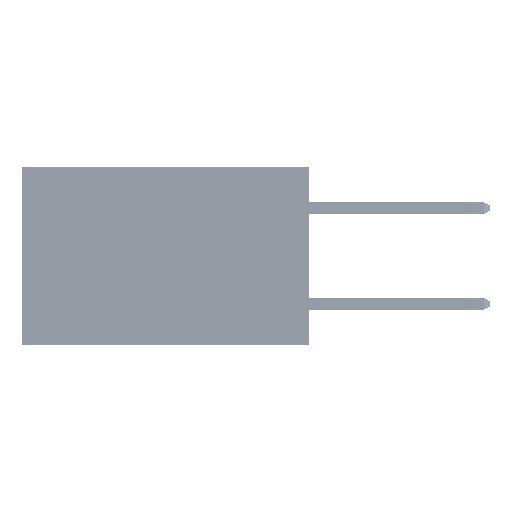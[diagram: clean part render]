
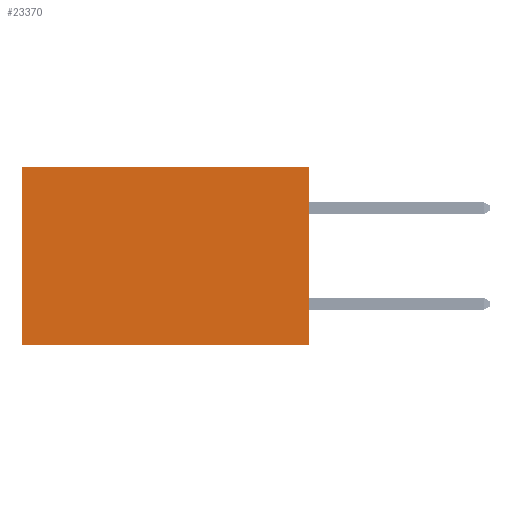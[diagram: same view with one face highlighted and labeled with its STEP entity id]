
A CAD part, left-side view. The second image highlights one B-rep face of the part: STEP entity #23370.
In plain terms, the highlighted planar face has unit normal (-1, 0, 0).
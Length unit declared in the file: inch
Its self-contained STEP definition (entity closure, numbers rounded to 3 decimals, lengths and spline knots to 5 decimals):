
#3877 = CARTESIAN_POINT ( 'NONE',  ( 0.2875, 0., 0. ) ) ;
#4240 = EDGE_CURVE ( 'NONE', #31126, #8284, #42876, .T. ) ;
#6278 = ORIENTED_EDGE ( 'NONE', *, *, #15349, .F. ) ;
#8284 = VERTEX_POINT ( 'NONE', #21485 ) ;
#8937 = VERTEX_POINT ( 'NONE', #30528 ) ;
#10186 = EDGE_LOOP ( 'NONE', ( #36949, #6278, #23037, #30390 ) ) ;
#10189 = CARTESIAN_POINT ( 'NONE',  ( 0.2875, 0.6, 0. ) ) ;
#12075 = AXIS2_PLACEMENT_3D ( 'NONE', #41348, #17093, #37240 ) ;
#12140 = VECTOR ( 'NONE', #31853, 39.37008 ) ;
#14491 = VECTOR ( 'NONE', #31919, 39.37008 ) ;
#15349 = EDGE_CURVE ( 'NONE', #8284, #30397, #39154, .T. ) ;
#16026 = CARTESIAN_POINT ( 'NONE',  ( 0.2875, 0., 0. ) ) ;
#17093 = DIRECTION ( 'NONE',  ( 1., 0., 0. ) ) ;
#17377 = VECTOR ( 'NONE', #38400, 39.37008 ) ;
#19308 = DIRECTION ( 'NONE',  ( 0., 0., -1. ) ) ;
#21485 = CARTESIAN_POINT ( 'NONE',  ( 0.2875, 0., -0.37 ) ) ;
#23037 = ORIENTED_EDGE ( 'NONE', *, *, #4240, .F. ) ;
#23370 = ADVANCED_FACE ( 'NONE', ( #31861 ), #48587, .F. ) ;
#27455 = CARTESIAN_POINT ( 'NONE',  ( 0.2875, 0.6, -0.37 ) ) ;
#28071 = LINE ( 'NONE', #3877, #12140 ) ;
#29906 = EDGE_CURVE ( 'NONE', #31126, #8937, #28071, .T. ) ;
#30390 = ORIENTED_EDGE ( 'NONE', *, *, #29906, .T. ) ;
#30397 = VERTEX_POINT ( 'NONE', #27455 ) ;
#30528 = CARTESIAN_POINT ( 'NONE',  ( 0.2875, 0.6, 0. ) ) ;
#31126 = VERTEX_POINT ( 'NONE', #16026 ) ;
#31853 = DIRECTION ( 'NONE',  ( 0., 1., 0. ) ) ;
#31861 = FACE_OUTER_BOUND ( 'NONE', #10186, .T. ) ;
#31919 = DIRECTION ( 'NONE',  ( 0., 1., 0. ) ) ;
#34276 = VECTOR ( 'NONE', #19308, 39.37008 ) ;
#34912 = EDGE_CURVE ( 'NONE', #8937, #30397, #49419, .T. ) ;
#36949 = ORIENTED_EDGE ( 'NONE', *, *, #34912, .T. ) ;
#37240 = DIRECTION ( 'NONE',  ( 0., 0., -1. ) ) ;
#38400 = DIRECTION ( 'NONE',  ( 0., 0., -1. ) ) ;
#39154 = LINE ( 'NONE', #39703, #14491 ) ;
#39703 = CARTESIAN_POINT ( 'NONE',  ( 0.2875, 0., -0.37 ) ) ;
#41348 = CARTESIAN_POINT ( 'NONE',  ( 0.2875, 0., 0. ) ) ;
#42876 = LINE ( 'NONE', #50826, #34276 ) ;
#48587 = PLANE ( 'NONE',  #12075 ) ;
#49419 = LINE ( 'NONE', #10189, #17377 ) ;
#50826 = CARTESIAN_POINT ( 'NONE',  ( 0.2875, 0., 0. ) ) ;
